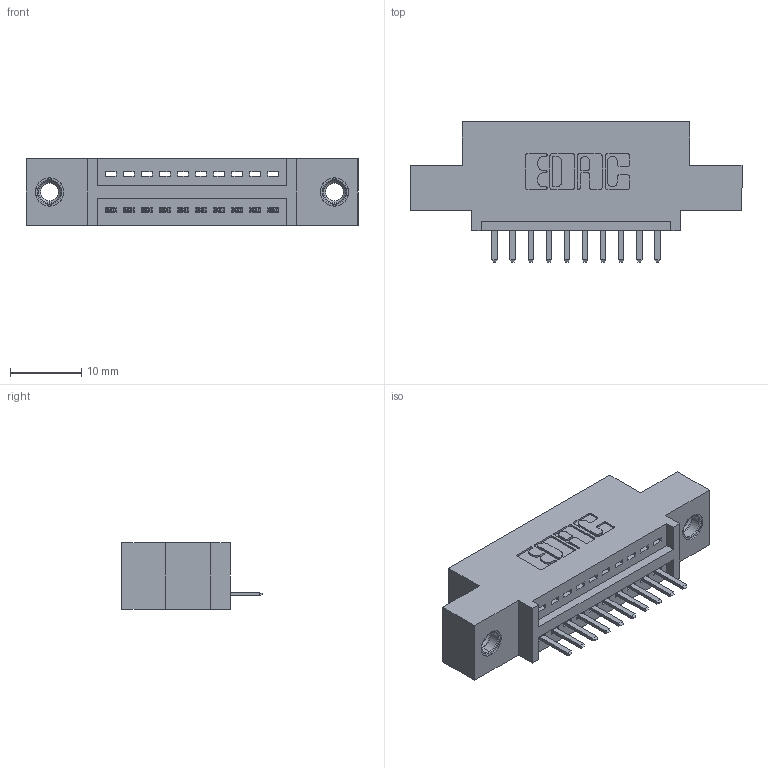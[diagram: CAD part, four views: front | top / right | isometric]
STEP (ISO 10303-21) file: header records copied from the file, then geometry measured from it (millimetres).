
FILE_DESCRIPTION (( 'STEP AP203' ), '1' );
FILE_NAME ('395-010-520-407.STEP', '2018-10-24T03:04:14', ( '' ), ( '' ), 'SwSTEP 2.0', 'SolidWorks 2016', '' );
FILE_SCHEMA (( 'CONFIG_CONTROL_DESIGN' ));
Length unit declared in the file: inch
Products named in the file (4): 345 Part_0.110 Offset - 0.156 Dia-TI; 345-292-001_345-293-120; 345-250-001_345-250-005-103; 395-010-520-407
Assembly tree (13 placements, depth 2):
  395-010-520-407
    345 Part_0.110 Offset - 0.156 Dia-TI
    345-292-001_345-293-120  x10
    345-250-001_345-250-005-103  x2
Bounding box: 46.61 x 19.68 x 9.4 mm (x, y, z)
Volume: 4049.2 mm3; surface area: 4966.4 mm2
Topology: 13 solids, 13 shells, 810 faces, 2329 edges, 1518 vertices
Faces by surface type: plane 536, cylinder 258, cone 12, torus 4
Entity records: 13266 total; most frequent: CARTESIAN_POINT 2293, ORIENTED_EDGE 2218, DIRECTION 2063, EDGE_CURVE 1109, LINE 913, VECTOR 913, VERTEX_POINT 732, AXIS2_PLACEMENT_3D 575
